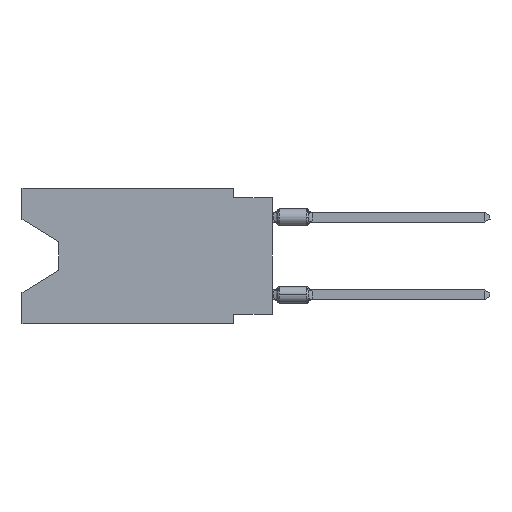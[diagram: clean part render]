
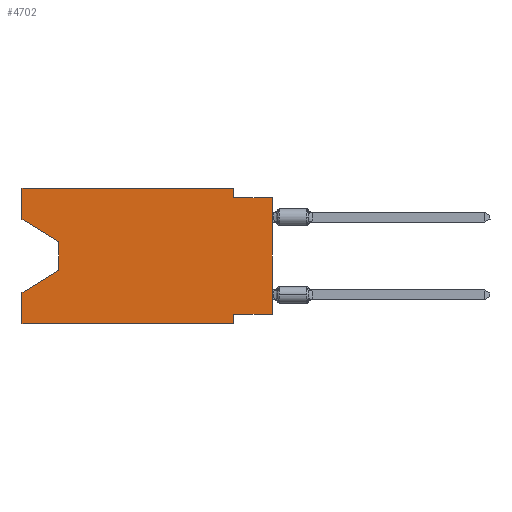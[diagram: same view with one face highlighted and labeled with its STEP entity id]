
A CAD part, left-side view. The second image highlights one B-rep face of the part: STEP entity #4702.
In plain terms, the highlighted planar face has unit normal (-1, 0, 0).
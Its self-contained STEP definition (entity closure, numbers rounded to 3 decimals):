
#40 = EDGE_CURVE ( 'NONE', #25245, #35237, #19683, .T. ) ;
#41 = CARTESIAN_POINT ( 'NONE',  ( 0., 16.383, 0. ) ) ;
#410 = DIRECTION ( 'NONE',  ( 0., 0., -1. ) ) ;
#1308 = EDGE_CURVE ( 'NONE', #7164, #33170, #11369, .T. ) ;
#1542 = EDGE_CURVE ( 'NONE', #47883, #27456, #34333, .T. ) ;
#2668 = DIRECTION ( 'NONE',  ( 0., -1., 0. ) ) ;
#3441 = CARTESIAN_POINT ( 'NONE',  ( 0., 13.97, -3.505 ) ) ;
#4414 = VERTEX_POINT ( 'NONE', #7635 ) ;
#4616 = VECTOR ( 'NONE', #42834, 1000. ) ;
#4702 = ADVANCED_FACE ( 'NONE', ( #7754 ), #38712, .F. ) ;
#5258 = VERTEX_POINT ( 'NONE', #41991 ) ;
#5364 = DIRECTION ( 'NONE',  ( 0., -0.855, -0.519 ) ) ;
#5707 = EDGE_CURVE ( 'NONE', #47883, #33170, #42415, .T. ) ;
#6339 = VECTOR ( 'NONE', #5364, 1000. ) ;
#7164 = VERTEX_POINT ( 'NONE', #25526 ) ;
#7385 = CARTESIAN_POINT ( 'NONE',  ( 0., 0., 0. ) ) ;
#7557 = VECTOR ( 'NONE', #25401, 1000. ) ;
#7635 = CARTESIAN_POINT ( 'NONE',  ( 0., 16.383, -8.89 ) ) ;
#7754 = FACE_OUTER_BOUND ( 'NONE', #22040, .T. ) ;
#8805 = ORIENTED_EDGE ( 'NONE', *, *, #21699, .F. ) ;
#9274 = ORIENTED_EDGE ( 'NONE', *, *, #18259, .F. ) ;
#9470 = LINE ( 'NONE', #32707, #6339 ) ;
#9563 = LINE ( 'NONE', #13893, #7557 ) ;
#10769 = DIRECTION ( 'NONE',  ( 0., 0.855, -0.519 ) ) ;
#11369 = LINE ( 'NONE', #26975, #4616 ) ;
#11955 = VECTOR ( 'NONE', #30500, 1000. ) ;
#13001 = EDGE_CURVE ( 'NONE', #4414, #5258, #33610, .T. ) ;
#13893 = CARTESIAN_POINT ( 'NONE',  ( 0., 16.383, 0. ) ) ;
#14775 = CARTESIAN_POINT ( 'NONE',  ( 0., 13.97, -3.505 ) ) ;
#14996 = VERTEX_POINT ( 'NONE', #32478 ) ;
#15955 = ORIENTED_EDGE ( 'NONE', *, *, #1542, .F. ) ;
#16000 = LINE ( 'NONE', #28497, #40130 ) ;
#16554 = CARTESIAN_POINT ( 'NONE',  ( 0., 16.383, -6.852 ) ) ;
#17044 = CARTESIAN_POINT ( 'NONE',  ( 0., 13.97, -5.385 ) ) ;
#17162 = CARTESIAN_POINT ( 'NONE',  ( 0., 16.383, 0. ) ) ;
#17637 = ORIENTED_EDGE ( 'NONE', *, *, #21564, .F. ) ;
#18252 = ORIENTED_EDGE ( 'NONE', *, *, #29650, .T. ) ;
#18259 = EDGE_CURVE ( 'NONE', #14996, #44939, #9563, .T. ) ;
#19201 = CARTESIAN_POINT ( 'NONE',  ( 0., 13.97, -5.385 ) ) ;
#19300 = EDGE_CURVE ( 'NONE', #32563, #7164, #23700, .T. ) ;
#19683 = LINE ( 'NONE', #19201, #44146 ) ;
#20849 = DIRECTION ( 'NONE',  ( 0., 0., -1. ) ) ;
#21335 = VECTOR ( 'NONE', #22852, 1000. ) ;
#21564 = EDGE_CURVE ( 'NONE', #27456, #5258, #16000, .T. ) ;
#21699 = EDGE_CURVE ( 'NONE', #4414, #35237, #38200, .T. ) ;
#21721 = VECTOR ( 'NONE', #2668, 1000. ) ;
#22040 = EDGE_LOOP ( 'NONE', ( #18252, #44295, #29528, #8805, #40902, #17637, #15955, #48590, #32349, #40026, #27207, #9274 ) ) ;
#22852 = DIRECTION ( 'NONE',  ( 0., 0., 1. ) ) ;
#22999 = DIRECTION ( 'NONE',  ( 0., 0., 1. ) ) ;
#23700 = LINE ( 'NONE', #39044, #38675 ) ;
#25245 = VERTEX_POINT ( 'NONE', #17044 ) ;
#25401 = DIRECTION ( 'NONE',  ( 0., 0., 1. ) ) ;
#25526 = CARTESIAN_POINT ( 'NONE',  ( 0., 2.54, -0.635 ) ) ;
#26298 = LINE ( 'NONE', #14775, #45930 ) ;
#26975 = CARTESIAN_POINT ( 'NONE',  ( 0., 0., -0.635 ) ) ;
#27207 = ORIENTED_EDGE ( 'NONE', *, *, #32018, .F. ) ;
#27456 = VERTEX_POINT ( 'NONE', #38150 ) ;
#28497 = CARTESIAN_POINT ( 'NONE',  ( 0., 2.54, -8.89 ) ) ;
#29528 = ORIENTED_EDGE ( 'NONE', *, *, #40, .T. ) ;
#29650 = EDGE_CURVE ( 'NONE', #14996, #44587, #9470, .T. ) ;
#30500 = DIRECTION ( 'NONE',  ( 0., 1., 0. ) ) ;
#32018 = EDGE_CURVE ( 'NONE', #44939, #32563, #36093, .T. ) ;
#32349 = ORIENTED_EDGE ( 'NONE', *, *, #1308, .F. ) ;
#32478 = CARTESIAN_POINT ( 'NONE',  ( 0., 16.383, -2.038 ) ) ;
#32563 = VERTEX_POINT ( 'NONE', #37302 ) ;
#32707 = CARTESIAN_POINT ( 'NONE',  ( 0., 16.383, -2.038 ) ) ;
#33170 = VERTEX_POINT ( 'NONE', #47383 ) ;
#33610 = LINE ( 'NONE', #49266, #21721 ) ;
#34333 = LINE ( 'NONE', #49995, #11955 ) ;
#35237 = VERTEX_POINT ( 'NONE', #16554 ) ;
#36093 = LINE ( 'NONE', #17162, #48179 ) ;
#36406 = EDGE_CURVE ( 'NONE', #44587, #25245, #26298, .T. ) ;
#37302 = CARTESIAN_POINT ( 'NONE',  ( 0., 2.54, 0. ) ) ;
#38150 = CARTESIAN_POINT ( 'NONE',  ( 0., 2.54, -8.255 ) ) ;
#38200 = LINE ( 'NONE', #49520, #21335 ) ;
#38675 = VECTOR ( 'NONE', #410, 1000. ) ;
#38712 = PLANE ( 'NONE',  #45028 ) ;
#39044 = CARTESIAN_POINT ( 'NONE',  ( 0., 2.54, 0. ) ) ;
#39382 = CARTESIAN_POINT ( 'NONE',  ( 0., 16.383, 0. ) ) ;
#40026 = ORIENTED_EDGE ( 'NONE', *, *, #19300, .F. ) ;
#40130 = VECTOR ( 'NONE', #20849, 1000. ) ;
#40902 = ORIENTED_EDGE ( 'NONE', *, *, #13001, .T. ) ;
#41890 = DIRECTION ( 'NONE',  ( 0., 0., -1. ) ) ;
#41894 = CARTESIAN_POINT ( 'NONE',  ( 0., 0., -8.255 ) ) ;
#41991 = CARTESIAN_POINT ( 'NONE',  ( 0., 2.54, -8.89 ) ) ;
#42415 = LINE ( 'NONE', #7385, #44514 ) ;
#42834 = DIRECTION ( 'NONE',  ( 0., -1., 0. ) ) ;
#43032 = DIRECTION ( 'NONE',  ( 0., 0., -1. ) ) ;
#44146 = VECTOR ( 'NONE', #10769, 1000. ) ;
#44295 = ORIENTED_EDGE ( 'NONE', *, *, #36406, .T. ) ;
#44514 = VECTOR ( 'NONE', #22999, 1000. ) ;
#44587 = VERTEX_POINT ( 'NONE', #3441 ) ;
#44939 = VERTEX_POINT ( 'NONE', #39382 ) ;
#45028 = AXIS2_PLACEMENT_3D ( 'NONE', #41, #46642, #43032 ) ;
#45050 = DIRECTION ( 'NONE',  ( 0., -1., 0. ) ) ;
#45930 = VECTOR ( 'NONE', #41890, 1000. ) ;
#46642 = DIRECTION ( 'NONE',  ( 1., 0., 0. ) ) ;
#47383 = CARTESIAN_POINT ( 'NONE',  ( 0., 0., -0.635 ) ) ;
#47883 = VERTEX_POINT ( 'NONE', #41894 ) ;
#48179 = VECTOR ( 'NONE', #45050, 1000. ) ;
#48590 = ORIENTED_EDGE ( 'NONE', *, *, #5707, .T. ) ;
#49266 = CARTESIAN_POINT ( 'NONE',  ( 0., 16.383, -8.89 ) ) ;
#49520 = CARTESIAN_POINT ( 'NONE',  ( 0., 16.383, 0. ) ) ;
#49995 = CARTESIAN_POINT ( 'NONE',  ( 0., 0., -8.255 ) ) ;
